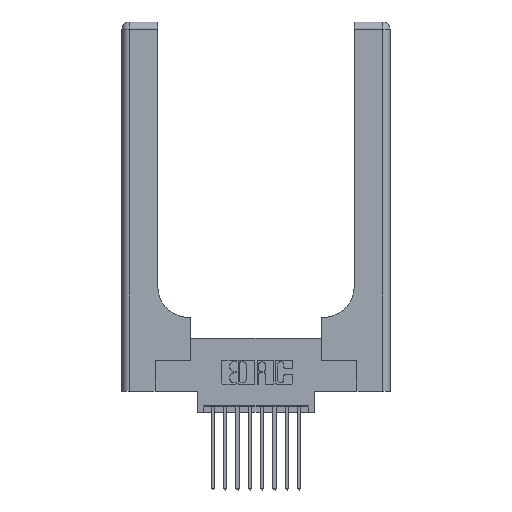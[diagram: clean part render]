
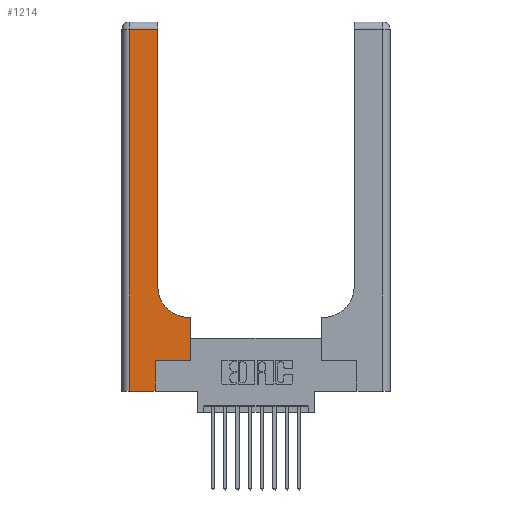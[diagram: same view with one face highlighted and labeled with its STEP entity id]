
A CAD part, top view. The second image highlights one B-rep face of the part: STEP entity #1214.
In plain terms, the highlighted planar face has unit normal (0, 0, 1).
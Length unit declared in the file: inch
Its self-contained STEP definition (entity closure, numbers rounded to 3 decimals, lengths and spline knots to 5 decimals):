
#94 = ORIENTED_EDGE ( 'NONE', *, *, #11444, .T. ) ;
#221 = CARTESIAN_POINT ( 'NONE',  ( 0.5415, 0.85, 0.37 ) ) ;
#236 = CARTESIAN_POINT ( 'NONE',  ( 0., 0., 0.37 ) ) ;
#403 = LINE ( 'NONE', #236, #7093 ) ;
#759 = VERTEX_POINT ( 'NONE', #7380 ) ;
#1166 = EDGE_CURVE ( 'NONE', #14751, #13248, #8195, .T. ) ;
#1214 = ADVANCED_FACE ( 'NONE', ( #4448 ), #14873, .F. ) ;
#1338 = VERTEX_POINT ( 'NONE', #13928 ) ;
#1352 = EDGE_CURVE ( 'NONE', #13248, #6272, #9158, .T. ) ;
#1477 = ORIENTED_EDGE ( 'NONE', *, *, #5161, .T. ) ;
#1497 = DIRECTION ( 'NONE',  ( 1., 0., 0. ) ) ;
#1513 = DIRECTION ( 'NONE',  ( 1., 0., 0. ) ) ;
#1617 = VECTOR ( 'NONE', #9018, 39.37008 ) ;
#2478 = ORIENTED_EDGE ( 'NONE', *, *, #4614, .T. ) ;
#2791 = CIRCLE ( 'NONE', #12257, 0.25 ) ;
#2962 = ORIENTED_EDGE ( 'NONE', *, *, #1166, .T. ) ;
#3949 = CARTESIAN_POINT ( 'NONE',  ( 0.5585, 0.25, 0.37 ) ) ;
#3970 = CARTESIAN_POINT ( 'NONE',  ( 0.269, 0., 0.37 ) ) ;
#4149 = DIRECTION ( 'NONE',  ( 0., -1., 0. ) ) ;
#4448 = FACE_OUTER_BOUND ( 'NONE', #7389, .T. ) ;
#4533 = AXIS2_PLACEMENT_3D ( 'NONE', #14859, #14808, #14790 ) ;
#4614 = EDGE_CURVE ( 'NONE', #6272, #1338, #5750, .T. ) ;
#4851 = VECTOR ( 'NONE', #15311, 39.37008 ) ;
#4948 = LINE ( 'NONE', #3970, #1617 ) ;
#5161 = EDGE_CURVE ( 'NONE', #5557, #8586, #4948, .T. ) ;
#5322 = CARTESIAN_POINT ( 'NONE',  ( 0.2915, 0.6, 0.37 ) ) ;
#5371 = CARTESIAN_POINT ( 'NONE',  ( 0.5415, 0.6, 0.37 ) ) ;
#5557 = VERTEX_POINT ( 'NONE', #15042 ) ;
#5639 = VECTOR ( 'NONE', #14051, 39.37008 ) ;
#5750 = LINE ( 'NONE', #10386, #15685 ) ;
#6091 = EDGE_CURVE ( 'NONE', #759, #12250, #15528, .T. ) ;
#6272 = VERTEX_POINT ( 'NONE', #8117 ) ;
#7093 = VECTOR ( 'NONE', #1513, 39.37008 ) ;
#7295 = EDGE_CURVE ( 'NONE', #13038, #14751, #2791, .T. ) ;
#7380 = CARTESIAN_POINT ( 'NONE',  ( 0.5585, 0.25, 0.37 ) ) ;
#7389 = EDGE_LOOP ( 'NONE', ( #2962, #10308, #2478, #8034, #1477, #11929, #12705, #94, #9647 ) ) ;
#7854 = DIRECTION ( 'NONE',  ( 0., 1., 0. ) ) ;
#8034 = ORIENTED_EDGE ( 'NONE', *, *, #13837, .T. ) ;
#8117 = CARTESIAN_POINT ( 'NONE',  ( 0.06, 2.94, 0.37 ) ) ;
#8195 = LINE ( 'NONE', #15626, #4851 ) ;
#8586 = VERTEX_POINT ( 'NONE', #8842 ) ;
#8594 = LINE ( 'NONE', #5322, #5639 ) ;
#8842 = CARTESIAN_POINT ( 'NONE',  ( 0.269, 0.25, 0.37 ) ) ;
#9006 = DIRECTION ( 'NONE',  ( 0., 0., -1. ) ) ;
#9018 = DIRECTION ( 'NONE',  ( 0., 1., 0. ) ) ;
#9158 = LINE ( 'NONE', #13646, #15381 ) ;
#9306 = VECTOR ( 'NONE', #7854, 39.37008 ) ;
#9512 = CARTESIAN_POINT ( 'NONE',  ( 0.5585, 0.6, 0.37 ) ) ;
#9647 = ORIENTED_EDGE ( 'NONE', *, *, #7295, .T. ) ;
#10208 = CARTESIAN_POINT ( 'NONE',  ( 0.269, 0.25, 0.37 ) ) ;
#10292 = LINE ( 'NONE', #10208, #16134 ) ;
#10308 = ORIENTED_EDGE ( 'NONE', *, *, #1352, .T. ) ;
#10386 = CARTESIAN_POINT ( 'NONE',  ( 0.06, 3., 0.37 ) ) ;
#11444 = EDGE_CURVE ( 'NONE', #12250, #13038, #8594, .T. ) ;
#11929 = ORIENTED_EDGE ( 'NONE', *, *, #12572, .T. ) ;
#12250 = VERTEX_POINT ( 'NONE', #9512 ) ;
#12257 = AXIS2_PLACEMENT_3D ( 'NONE', #221, #9006, #1497 ) ;
#12572 = EDGE_CURVE ( 'NONE', #8586, #759, #10292, .T. ) ;
#12705 = ORIENTED_EDGE ( 'NONE', *, *, #6091, .T. ) ;
#13038 = VERTEX_POINT ( 'NONE', #5371 ) ;
#13248 = VERTEX_POINT ( 'NONE', #14368 ) ;
#13646 = CARTESIAN_POINT ( 'NONE',  ( 0., 2.94, 0.37 ) ) ;
#13773 = DIRECTION ( 'NONE',  ( -1., 0., 0. ) ) ;
#13837 = EDGE_CURVE ( 'NONE', #1338, #5557, #403, .T. ) ;
#13928 = CARTESIAN_POINT ( 'NONE',  ( 0.06, 0., 0.37 ) ) ;
#14051 = DIRECTION ( 'NONE',  ( -1., 0., 0. ) ) ;
#14368 = CARTESIAN_POINT ( 'NONE',  ( 0.2915, 2.94, 0.37 ) ) ;
#14710 = CARTESIAN_POINT ( 'NONE',  ( 0.2915, 0.85, 0.37 ) ) ;
#14751 = VERTEX_POINT ( 'NONE', #14710 ) ;
#14790 = DIRECTION ( 'NONE',  ( -1., 0., 0. ) ) ;
#14808 = DIRECTION ( 'NONE',  ( 0., 0., -1. ) ) ;
#14859 = CARTESIAN_POINT ( 'NONE',  ( 0., 3., 0.37 ) ) ;
#14873 = PLANE ( 'NONE',  #4533 ) ;
#15042 = CARTESIAN_POINT ( 'NONE',  ( 0.269, 0., 0.37 ) ) ;
#15212 = DIRECTION ( 'NONE',  ( 1., 0., 0. ) ) ;
#15311 = DIRECTION ( 'NONE',  ( 0., 1., 0. ) ) ;
#15381 = VECTOR ( 'NONE', #13773, 39.37008 ) ;
#15528 = LINE ( 'NONE', #3949, #9306 ) ;
#15626 = CARTESIAN_POINT ( 'NONE',  ( 0.2915, 3., 0.37 ) ) ;
#15685 = VECTOR ( 'NONE', #4149, 39.37008 ) ;
#16134 = VECTOR ( 'NONE', #15212, 39.37008 ) ;
